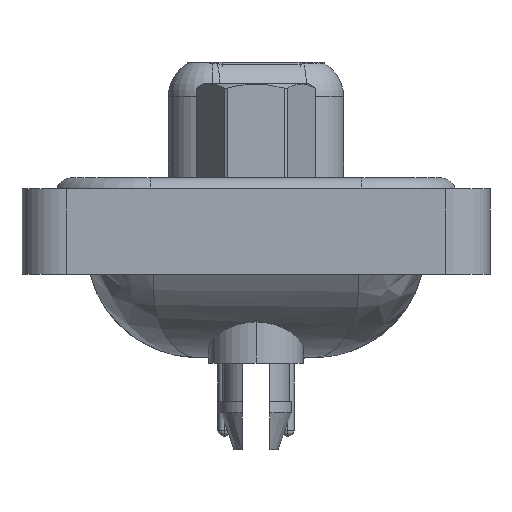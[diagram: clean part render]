
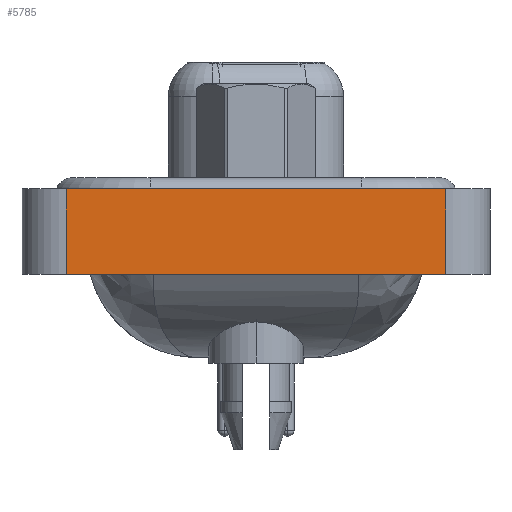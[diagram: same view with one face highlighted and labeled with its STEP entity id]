
A CAD part, left-side view. The second image highlights one B-rep face of the part: STEP entity #5785.
In plain terms, the highlighted planar face has unit normal (-1, 0, 0).
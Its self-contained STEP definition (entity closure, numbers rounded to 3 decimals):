
#485 = EDGE_CURVE ( 'NONE', #22155, #6361, #11085, .T. ) ;
#2445 = DIRECTION ( 'NONE',  ( -1., 0., 0. ) ) ;
#2637 = CARTESIAN_POINT ( 'NONE',  ( -7.25, -8.55, -3.35 ) ) ;
#2936 = EDGE_LOOP ( 'NONE', ( #14778, #3974, #3921, #7005 ) ) ;
#3718 = LINE ( 'NONE', #17024, #19335 ) ;
#3921 = ORIENTED_EDGE ( 'NONE', *, *, #16551, .F. ) ;
#3974 = ORIENTED_EDGE ( 'NONE', *, *, #5799, .F. ) ;
#3989 = CARTESIAN_POINT ( 'NONE',  ( -7.25, 8.55, -3.35 ) ) ;
#4139 = LINE ( 'NONE', #9830, #17145 ) ;
#4348 = LINE ( 'NONE', #2637, #10246 ) ;
#4829 = VERTEX_POINT ( 'NONE', #3989 ) ;
#5586 = CARTESIAN_POINT ( 'NONE',  ( -7.25, 8.55, 0.5 ) ) ;
#5703 = DIRECTION ( 'NONE',  ( 0., 0., 1. ) ) ;
#5785 = ADVANCED_FACE ( 'NONE', ( #18296 ), #20097, .T. ) ;
#5799 = EDGE_CURVE ( 'NONE', #6556, #6361, #4139, .T. ) ;
#6361 = VERTEX_POINT ( 'NONE', #8300 ) ;
#6556 = VERTEX_POINT ( 'NONE', #5586 ) ;
#7005 = ORIENTED_EDGE ( 'NONE', *, *, #12915, .T. ) ;
#8040 = CARTESIAN_POINT ( 'NONE',  ( -7.25, -8.55, -3.35 ) ) ;
#8157 = AXIS2_PLACEMENT_3D ( 'NONE', #8040, #2445, #16613 ) ;
#8300 = CARTESIAN_POINT ( 'NONE',  ( -7.25, -8.55, 0.5 ) ) ;
#9298 = DIRECTION ( 'NONE',  ( 0., -1., 0. ) ) ;
#9830 = CARTESIAN_POINT ( 'NONE',  ( -7.25, -8.55, 0.5 ) ) ;
#10246 = VECTOR ( 'NONE', #9298, 1000. ) ;
#10595 = DIRECTION ( 'NONE',  ( 0., 0., 1. ) ) ;
#11085 = LINE ( 'NONE', #19664, #14949 ) ;
#12915 = EDGE_CURVE ( 'NONE', #4829, #22155, #4348, .T. ) ;
#13109 = DIRECTION ( 'NONE',  ( 0., -1., 0. ) ) ;
#14778 = ORIENTED_EDGE ( 'NONE', *, *, #485, .T. ) ;
#14949 = VECTOR ( 'NONE', #5703, 1000. ) ;
#16551 = EDGE_CURVE ( 'NONE', #4829, #6556, #3718, .T. ) ;
#16613 = DIRECTION ( 'NONE',  ( 0., 0., 1. ) ) ;
#17024 = CARTESIAN_POINT ( 'NONE',  ( -7.25, 8.55, -3.35 ) ) ;
#17145 = VECTOR ( 'NONE', #13109, 1000. ) ;
#18296 = FACE_OUTER_BOUND ( 'NONE', #2936, .T. ) ;
#19335 = VECTOR ( 'NONE', #10595, 1000. ) ;
#19664 = CARTESIAN_POINT ( 'NONE',  ( -7.25, -8.55, -3.35 ) ) ;
#19796 = CARTESIAN_POINT ( 'NONE',  ( -7.25, -8.55, -3.35 ) ) ;
#20097 = PLANE ( 'NONE',  #8157 ) ;
#22155 = VERTEX_POINT ( 'NONE', #19796 ) ;
